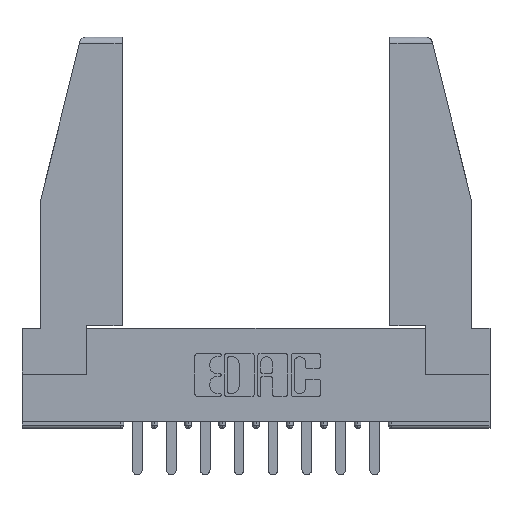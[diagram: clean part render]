
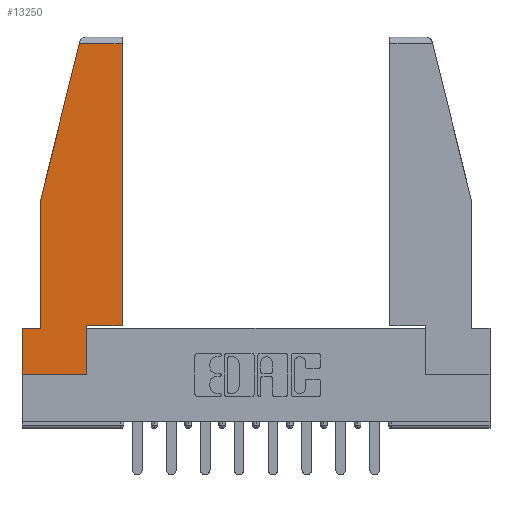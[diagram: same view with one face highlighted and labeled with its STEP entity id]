
A CAD part, top view. The second image highlights one B-rep face of the part: STEP entity #13250.
In plain terms, the highlighted planar face has unit normal (0, 0, 1).
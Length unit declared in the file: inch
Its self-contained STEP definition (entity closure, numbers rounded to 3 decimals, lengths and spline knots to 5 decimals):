
#101 = CARTESIAN_POINT ( 'NONE',  ( 0.461, 1.52, 0. ) ) ;
#404 = ORIENTED_EDGE ( 'NONE', *, *, #12013, .T. ) ;
#621 = VERTEX_POINT ( 'NONE', #7770 ) ;
#1088 = EDGE_CURVE ( 'NONE', #12506, #12721, #11711, .T. ) ;
#1101 = CARTESIAN_POINT ( 'NONE',  ( 0.297, 0.223, 0. ) ) ;
#1205 = CARTESIAN_POINT ( 'NONE',  ( 0.461, 0.223, 0. ) ) ;
#1439 = CARTESIAN_POINT ( 'NONE',  ( 0.297, 0., 0. ) ) ;
#1604 = VECTOR ( 'NONE', #7090, 39.37008 ) ;
#2121 = DIRECTION ( 'NONE',  ( 0., -1., 0. ) ) ;
#2180 = CARTESIAN_POINT ( 'NONE',  ( 0.086, 0.8, 0. ) ) ;
#2310 = EDGE_CURVE ( 'NONE', #10911, #10519, #2336, .T. ) ;
#2336 = LINE ( 'NONE', #9545, #1604 ) ;
#2508 = CARTESIAN_POINT ( 'NONE',  ( 0.2636, 1.52, 0. ) ) ;
#2554 = LINE ( 'NONE', #2180, #11166 ) ;
#2951 = DIRECTION ( 'NONE',  ( 0., 1., 0. ) ) ;
#3030 = ORIENTED_EDGE ( 'NONE', *, *, #9926, .T. ) ;
#3585 = FACE_OUTER_BOUND ( 'NONE', #14436, .T. ) ;
#3799 = DIRECTION ( 'NONE',  ( 0., 1., 0. ) ) ;
#4532 = DIRECTION ( 'NONE',  ( 1., 0., 0. ) ) ;
#4536 = DIRECTION ( 'NONE',  ( 1., 0., 0. ) ) ;
#4745 = EDGE_CURVE ( 'NONE', #7976, #12506, #8159, .T. ) ;
#5117 = ORIENTED_EDGE ( 'NONE', *, *, #4745, .T. ) ;
#5343 = LINE ( 'NONE', #1101, #13183 ) ;
#6431 = DIRECTION ( 'NONE',  ( -0.239, -0.971, 0. ) ) ;
#6579 = CARTESIAN_POINT ( 'NONE',  ( 0.297, 0., 0. ) ) ;
#6734 = VECTOR ( 'NONE', #9034, 39.37008 ) ;
#6941 = PLANE ( 'NONE',  #9197 ) ;
#7017 = LINE ( 'NONE', #9842, #13963 ) ;
#7090 = DIRECTION ( 'NONE',  ( -1., 0., 0. ) ) ;
#7243 = CARTESIAN_POINT ( 'NONE',  ( 0., 0.21, 0. ) ) ;
#7479 = ORIENTED_EDGE ( 'NONE', *, *, #14193, .T. ) ;
#7770 = CARTESIAN_POINT ( 'NONE',  ( 0.086, 0.21, 0. ) ) ;
#7870 = EDGE_CURVE ( 'NONE', #10519, #11054, #7017, .T. ) ;
#7976 = VERTEX_POINT ( 'NONE', #14874 ) ;
#8120 = DIRECTION ( 'NONE',  ( 1., 0., 0. ) ) ;
#8159 = LINE ( 'NONE', #12843, #8878 ) ;
#8878 = VECTOR ( 'NONE', #4536, 39.37008 ) ;
#9034 = DIRECTION ( 'NONE',  ( -1., 0., 0. ) ) ;
#9197 = AXIS2_PLACEMENT_3D ( 'NONE', #14021, #10508, #8120 ) ;
#9367 = VECTOR ( 'NONE', #13016, 39.37008 ) ;
#9510 = EDGE_CURVE ( 'NONE', #13512, #7976, #9738, .T. ) ;
#9545 = CARTESIAN_POINT ( 'NONE',  ( 0., 1.52, 0. ) ) ;
#9692 = LINE ( 'NONE', #11031, #10425 ) ;
#9738 = LINE ( 'NONE', #7243, #9367 ) ;
#9767 = ORIENTED_EDGE ( 'NONE', *, *, #9510, .T. ) ;
#9841 = ORIENTED_EDGE ( 'NONE', *, *, #1088, .T. ) ;
#9842 = CARTESIAN_POINT ( 'NONE',  ( 0.271, 1.55, 0. ) ) ;
#9926 = EDGE_CURVE ( 'NONE', #12721, #12130, #5343, .T. ) ;
#9968 = ORIENTED_EDGE ( 'NONE', *, *, #2310, .T. ) ;
#10425 = VECTOR ( 'NONE', #2951, 39.37008 ) ;
#10508 = DIRECTION ( 'NONE',  ( 0., 0., 1. ) ) ;
#10519 = VERTEX_POINT ( 'NONE', #2508 ) ;
#10911 = VERTEX_POINT ( 'NONE', #101 ) ;
#11031 = CARTESIAN_POINT ( 'NONE',  ( 0.461, 0.223, 0. ) ) ;
#11054 = VERTEX_POINT ( 'NONE', #11863 ) ;
#11166 = VECTOR ( 'NONE', #2121, 39.37008 ) ;
#11639 = ORIENTED_EDGE ( 'NONE', *, *, #7870, .T. ) ;
#11711 = LINE ( 'NONE', #1439, #14799 ) ;
#11863 = CARTESIAN_POINT ( 'NONE',  ( 0.086, 0.8, 0. ) ) ;
#12013 = EDGE_CURVE ( 'NONE', #621, #13512, #14560, .T. ) ;
#12130 = VERTEX_POINT ( 'NONE', #1205 ) ;
#12340 = ORIENTED_EDGE ( 'NONE', *, *, #14557, .T. ) ;
#12506 = VERTEX_POINT ( 'NONE', #6579 ) ;
#12721 = VERTEX_POINT ( 'NONE', #15109 ) ;
#12728 = CARTESIAN_POINT ( 'NONE',  ( 0., 0.21, 0. ) ) ;
#12843 = CARTESIAN_POINT ( 'NONE',  ( 0., 0., 0. ) ) ;
#13016 = DIRECTION ( 'NONE',  ( 0., -1., 0. ) ) ;
#13183 = VECTOR ( 'NONE', #4532, 39.37008 ) ;
#13250 = ADVANCED_FACE ( 'NONE', ( #3585 ), #6941, .T. ) ;
#13512 = VERTEX_POINT ( 'NONE', #12728 ) ;
#13672 = CARTESIAN_POINT ( 'NONE',  ( 0., 0.21, 0. ) ) ;
#13963 = VECTOR ( 'NONE', #6431, 39.37008 ) ;
#14021 = CARTESIAN_POINT ( 'NONE',  ( 0., 0., 0. ) ) ;
#14193 = EDGE_CURVE ( 'NONE', #11054, #621, #2554, .T. ) ;
#14436 = EDGE_LOOP ( 'NONE', ( #12340, #9968, #11639, #7479, #404, #9767, #5117, #9841, #3030 ) ) ;
#14557 = EDGE_CURVE ( 'NONE', #12130, #10911, #9692, .T. ) ;
#14560 = LINE ( 'NONE', #13672, #6734 ) ;
#14799 = VECTOR ( 'NONE', #3799, 39.37008 ) ;
#14874 = CARTESIAN_POINT ( 'NONE',  ( 0., 0., 0. ) ) ;
#15109 = CARTESIAN_POINT ( 'NONE',  ( 0.297, 0.223, 0. ) ) ;
